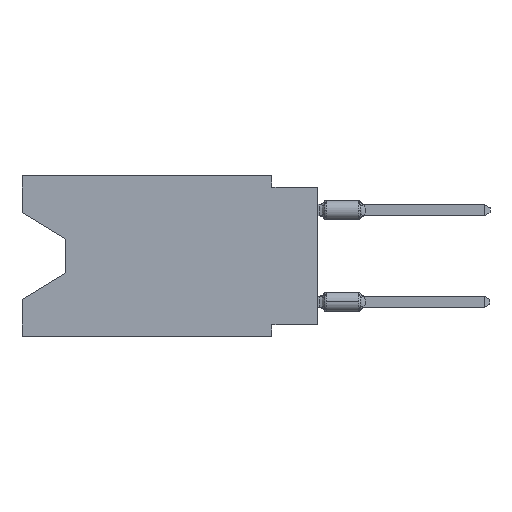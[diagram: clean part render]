
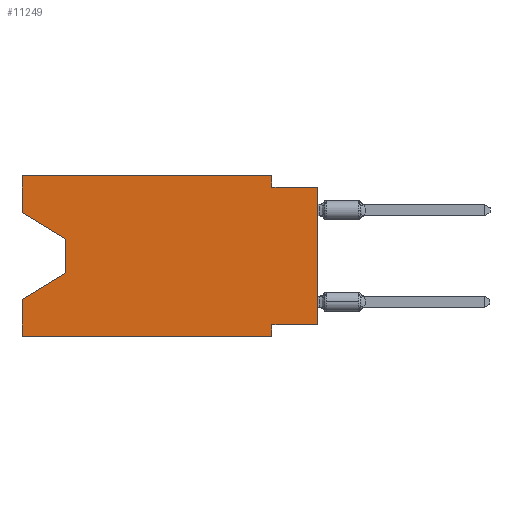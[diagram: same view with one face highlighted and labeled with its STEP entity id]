
A CAD part, left-side view. The second image highlights one B-rep face of the part: STEP entity #11249.
In plain terms, the highlighted planar face has unit normal (-1, 0, 0).
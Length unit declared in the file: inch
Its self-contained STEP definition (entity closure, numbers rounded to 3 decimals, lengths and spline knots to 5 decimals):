
#153 = VECTOR ( 'NONE', #20802, 39.37008 ) ;
#1207 = ORIENTED_EDGE ( 'NONE', *, *, #3569, .T. ) ;
#1903 = VERTEX_POINT ( 'NONE', #17201 ) ;
#2048 = ORIENTED_EDGE ( 'NONE', *, *, #24617, .F. ) ;
#2130 = CARTESIAN_POINT ( 'NONE',  ( 0., 0., -0.325 ) ) ;
#2330 = VERTEX_POINT ( 'NONE', #16781 ) ;
#2514 = VECTOR ( 'NONE', #24811, 39.37008 ) ;
#3055 = LINE ( 'NONE', #24032, #5162 ) ;
#3086 = DIRECTION ( 'NONE',  ( 0., 0., -1. ) ) ;
#3352 = VECTOR ( 'NONE', #36688, 39.37008 ) ;
#3569 = EDGE_CURVE ( 'NONE', #33642, #26587, #27039, .T. ) ;
#3811 = VERTEX_POINT ( 'NONE', #19077 ) ;
#3857 = VECTOR ( 'NONE', #33735, 39.37008 ) ;
#4302 = EDGE_CURVE ( 'NONE', #1903, #35879, #8256, .T. ) ;
#4978 = EDGE_CURVE ( 'NONE', #32879, #10029, #37272, .T. ) ;
#5162 = VECTOR ( 'NONE', #6281, 39.37008 ) ;
#5707 = ORIENTED_EDGE ( 'NONE', *, *, #18867, .T. ) ;
#6281 = DIRECTION ( 'NONE',  ( 0., -1., 0. ) ) ;
#6553 = CARTESIAN_POINT ( 'NONE',  ( 0., 0.645, 0. ) ) ;
#7424 = ORIENTED_EDGE ( 'NONE', *, *, #29876, .T. ) ;
#8095 = VECTOR ( 'NONE', #10137, 39.37008 ) ;
#8256 = LINE ( 'NONE', #31270, #3857 ) ;
#9365 = LINE ( 'NONE', #6553, #14438 ) ;
#10029 = VERTEX_POINT ( 'NONE', #28555 ) ;
#10137 = DIRECTION ( 'NONE',  ( 0., 0., 1. ) ) ;
#10206 = VERTEX_POINT ( 'NONE', #28754 ) ;
#10407 = ORIENTED_EDGE ( 'NONE', *, *, #36921, .F. ) ;
#10417 = PLANE ( 'NONE',  #18491 ) ;
#11249 = ADVANCED_FACE ( 'NONE', ( #19633 ), #10417, .F. ) ;
#11770 = DIRECTION ( 'NONE',  ( 0., -1., 0. ) ) ;
#12187 = CARTESIAN_POINT ( 'NONE',  ( 0., 0., -0.025 ) ) ;
#12677 = LINE ( 'NONE', #14752, #13661 ) ;
#13661 = VECTOR ( 'NONE', #26271, 39.37008 ) ;
#13848 = CARTESIAN_POINT ( 'NONE',  ( 0., 0.645, -0.26975 ) ) ;
#14009 = CARTESIAN_POINT ( 'NONE',  ( 0., 0.645, -0.08025 ) ) ;
#14438 = VECTOR ( 'NONE', #18051, 39.37008 ) ;
#14582 = LINE ( 'NONE', #32135, #22639 ) ;
#14605 = CARTESIAN_POINT ( 'NONE',  ( 0., 0.1, 0. ) ) ;
#14701 = ORIENTED_EDGE ( 'NONE', *, *, #37131, .F. ) ;
#14751 = EDGE_CURVE ( 'NONE', #35879, #32879, #9365, .T. ) ;
#14752 = CARTESIAN_POINT ( 'NONE',  ( 0., 0.55, -0.138 ) ) ;
#15513 = DIRECTION ( 'NONE',  ( 0., 0., 1. ) ) ;
#15526 = EDGE_CURVE ( 'NONE', #2330, #3811, #3055, .T. ) ;
#16781 = CARTESIAN_POINT ( 'NONE',  ( 0., 0.645, -0.35 ) ) ;
#16832 = ORIENTED_EDGE ( 'NONE', *, *, #15526, .T. ) ;
#17201 = CARTESIAN_POINT ( 'NONE',  ( 0., 0.645, -0.08025 ) ) ;
#17582 = ORIENTED_EDGE ( 'NONE', *, *, #4978, .F. ) ;
#18051 = DIRECTION ( 'NONE',  ( 0., -1., 0. ) ) ;
#18332 = LINE ( 'NONE', #34813, #26614 ) ;
#18491 = AXIS2_PLACEMENT_3D ( 'NONE', #27404, #33428, #36092 ) ;
#18867 = EDGE_CURVE ( 'NONE', #10206, #25040, #18332, .T. ) ;
#19077 = CARTESIAN_POINT ( 'NONE',  ( 0., 0.1, -0.35 ) ) ;
#19633 = FACE_OUTER_BOUND ( 'NONE', #31660, .T. ) ;
#20802 = DIRECTION ( 'NONE',  ( 0., 0.855, -0.519 ) ) ;
#21811 = CARTESIAN_POINT ( 'NONE',  ( 0., 0.645, 0. ) ) ;
#22106 = CARTESIAN_POINT ( 'NONE',  ( 0., 0.1, -0.325 ) ) ;
#22187 = DIRECTION ( 'NONE',  ( 0., 0., -1. ) ) ;
#22639 = VECTOR ( 'NONE', #11770, 39.37008 ) ;
#22730 = LINE ( 'NONE', #30846, #33429 ) ;
#24032 = CARTESIAN_POINT ( 'NONE',  ( 0., 0.645, -0.35 ) ) ;
#24617 = EDGE_CURVE ( 'NONE', #2330, #26587, #24660, .T. ) ;
#24660 = LINE ( 'NONE', #21811, #8095 ) ;
#24811 = DIRECTION ( 'NONE',  ( 0., -0.855, -0.519 ) ) ;
#25040 = VERTEX_POINT ( 'NONE', #12187 ) ;
#25143 = ORIENTED_EDGE ( 'NONE', *, *, #26586, .F. ) ;
#25938 = CARTESIAN_POINT ( 'NONE',  ( 0., 0.55, -0.138 ) ) ;
#26271 = DIRECTION ( 'NONE',  ( 0., 0., -1. ) ) ;
#26586 = EDGE_CURVE ( 'NONE', #29052, #3811, #22730, .T. ) ;
#26587 = VERTEX_POINT ( 'NONE', #13848 ) ;
#26614 = VECTOR ( 'NONE', #15513, 39.37008 ) ;
#27039 = LINE ( 'NONE', #35137, #153 ) ;
#27404 = CARTESIAN_POINT ( 'NONE',  ( 0., 0.645, 0. ) ) ;
#27654 = LINE ( 'NONE', #2130, #3352 ) ;
#27661 = CARTESIAN_POINT ( 'NONE',  ( 0., 0.1, 0. ) ) ;
#28145 = VERTEX_POINT ( 'NONE', #25938 ) ;
#28185 = LINE ( 'NONE', #14009, #2514 ) ;
#28555 = CARTESIAN_POINT ( 'NONE',  ( 0., 0.1, -0.025 ) ) ;
#28587 = ORIENTED_EDGE ( 'NONE', *, *, #14751, .F. ) ;
#28747 = EDGE_CURVE ( 'NONE', #28145, #33642, #12677, .T. ) ;
#28754 = CARTESIAN_POINT ( 'NONE',  ( 0., 0., -0.325 ) ) ;
#29052 = VERTEX_POINT ( 'NONE', #22106 ) ;
#29876 = EDGE_CURVE ( 'NONE', #1903, #28145, #28185, .T. ) ;
#30846 = CARTESIAN_POINT ( 'NONE',  ( 0., 0.1, -0.35 ) ) ;
#31270 = CARTESIAN_POINT ( 'NONE',  ( 0., 0.645, 0. ) ) ;
#31660 = EDGE_LOOP ( 'NONE', ( #7424, #32782, #1207, #2048, #16832, #25143, #10407, #5707, #14701, #17582, #28587, #32558 ) ) ;
#32135 = CARTESIAN_POINT ( 'NONE',  ( 0., 0., -0.025 ) ) ;
#32558 = ORIENTED_EDGE ( 'NONE', *, *, #4302, .F. ) ;
#32782 = ORIENTED_EDGE ( 'NONE', *, *, #28747, .T. ) ;
#32879 = VERTEX_POINT ( 'NONE', #27661 ) ;
#33428 = DIRECTION ( 'NONE',  ( 1., 0., 0. ) ) ;
#33429 = VECTOR ( 'NONE', #22187, 39.37008 ) ;
#33642 = VERTEX_POINT ( 'NONE', #36242 ) ;
#33735 = DIRECTION ( 'NONE',  ( 0., 0., 1. ) ) ;
#34011 = VECTOR ( 'NONE', #3086, 39.37008 ) ;
#34797 = CARTESIAN_POINT ( 'NONE',  ( 0., 0.645, 0. ) ) ;
#34813 = CARTESIAN_POINT ( 'NONE',  ( 0., 0., 0. ) ) ;
#35137 = CARTESIAN_POINT ( 'NONE',  ( 0., 0.55, -0.212 ) ) ;
#35879 = VERTEX_POINT ( 'NONE', #34797 ) ;
#36092 = DIRECTION ( 'NONE',  ( 0., 0., -1. ) ) ;
#36242 = CARTESIAN_POINT ( 'NONE',  ( 0., 0.55, -0.212 ) ) ;
#36688 = DIRECTION ( 'NONE',  ( 0., 1., 0. ) ) ;
#36921 = EDGE_CURVE ( 'NONE', #10206, #29052, #27654, .T. ) ;
#37131 = EDGE_CURVE ( 'NONE', #10029, #25040, #14582, .T. ) ;
#37272 = LINE ( 'NONE', #14605, #34011 ) ;
